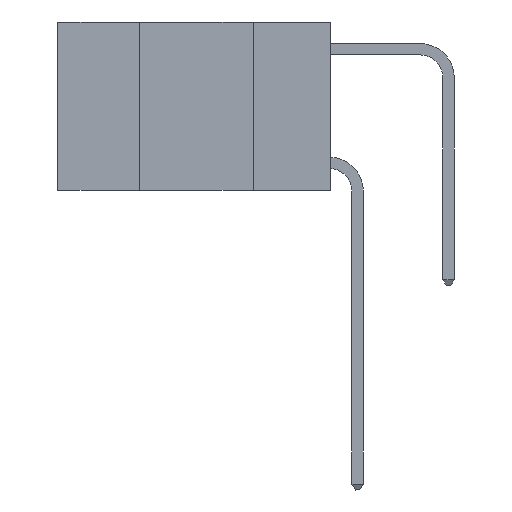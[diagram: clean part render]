
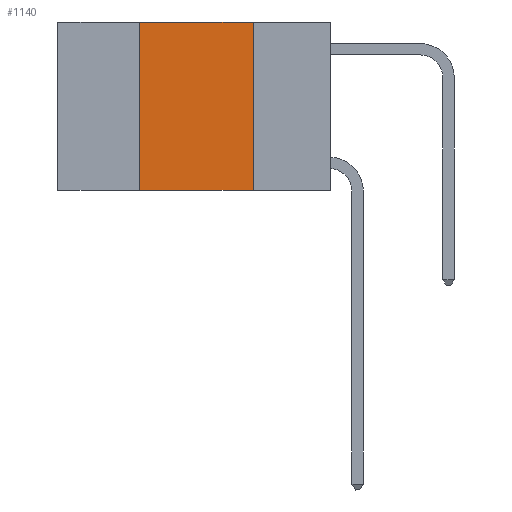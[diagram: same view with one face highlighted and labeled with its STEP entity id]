
A CAD part, left-side view. The second image highlights one B-rep face of the part: STEP entity #1140.
In plain terms, the highlighted planar face has unit normal (-1, 0, 0).
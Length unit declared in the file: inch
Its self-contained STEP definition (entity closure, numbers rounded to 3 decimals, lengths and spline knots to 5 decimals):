
#1140 = ADVANCED_FACE ( 'NONE', ( #29289 ), #4731, .F. ) ;
#1462 = DIRECTION ( 'NONE',  ( 0., -1., 0. ) ) ;
#1975 = CARTESIAN_POINT ( 'NONE',  ( 0., 0.42, -0.37 ) ) ;
#3993 = CARTESIAN_POINT ( 'NONE',  ( 0., 0.42, 0. ) ) ;
#4731 = PLANE ( 'NONE',  #4845 ) ;
#4845 = AXIS2_PLACEMENT_3D ( 'NONE', #9564, #22105, #7197 ) ;
#4964 = CARTESIAN_POINT ( 'NONE',  ( 0., 0.6, 0. ) ) ;
#6053 = VERTEX_POINT ( 'NONE', #1975 ) ;
#6189 = LINE ( 'NONE', #6783, #31078 ) ;
#6531 = EDGE_LOOP ( 'NONE', ( #24503, #26574, #28033, #28777 ) ) ;
#6783 = CARTESIAN_POINT ( 'NONE',  ( 0., 0.17, 0. ) ) ;
#7197 = DIRECTION ( 'NONE',  ( 0., 0., -1. ) ) ;
#9238 = DIRECTION ( 'NONE',  ( 0., 0., -1. ) ) ;
#9564 = CARTESIAN_POINT ( 'NONE',  ( 0., 0.6, 0. ) ) ;
#10390 = LINE ( 'NONE', #4964, #15471 ) ;
#10813 = VECTOR ( 'NONE', #31352, 39.37008 ) ;
#10915 = EDGE_CURVE ( 'NONE', #6053, #15382, #17495, .T. ) ;
#11602 = LINE ( 'NONE', #3993, #10813 ) ;
#12737 = EDGE_CURVE ( 'NONE', #15701, #15382, #6189, .T. ) ;
#14918 = DIRECTION ( 'NONE',  ( 0., -1., 0. ) ) ;
#15382 = VERTEX_POINT ( 'NONE', #25469 ) ;
#15471 = VECTOR ( 'NONE', #14918, 39.37008 ) ;
#15697 = VERTEX_POINT ( 'NONE', #31548 ) ;
#15701 = VERTEX_POINT ( 'NONE', #29077 ) ;
#17495 = LINE ( 'NONE', #31202, #23386 ) ;
#20478 = EDGE_CURVE ( 'NONE', #15697, #15701, #10390, .T. ) ;
#22105 = DIRECTION ( 'NONE',  ( 1., 0., 0. ) ) ;
#23386 = VECTOR ( 'NONE', #1462, 39.37008 ) ;
#24045 = EDGE_CURVE ( 'NONE', #6053, #15697, #11602, .T. ) ;
#24503 = ORIENTED_EDGE ( 'NONE', *, *, #12737, .F. ) ;
#25469 = CARTESIAN_POINT ( 'NONE',  ( 0., 0.17, -0.37 ) ) ;
#26574 = ORIENTED_EDGE ( 'NONE', *, *, #20478, .F. ) ;
#28033 = ORIENTED_EDGE ( 'NONE', *, *, #24045, .F. ) ;
#28777 = ORIENTED_EDGE ( 'NONE', *, *, #10915, .T. ) ;
#29077 = CARTESIAN_POINT ( 'NONE',  ( 0., 0.17, 0. ) ) ;
#29289 = FACE_OUTER_BOUND ( 'NONE', #6531, .T. ) ;
#31078 = VECTOR ( 'NONE', #9238, 39.37008 ) ;
#31202 = CARTESIAN_POINT ( 'NONE',  ( 0., 0.6, -0.37 ) ) ;
#31352 = DIRECTION ( 'NONE',  ( 0., 0., 1. ) ) ;
#31548 = CARTESIAN_POINT ( 'NONE',  ( 0., 0.42, 0. ) ) ;
